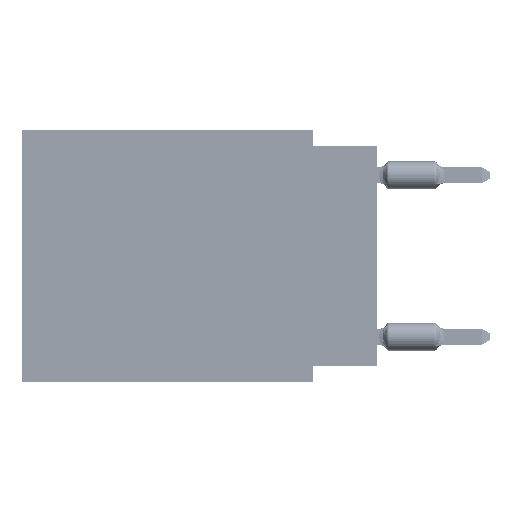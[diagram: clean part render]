
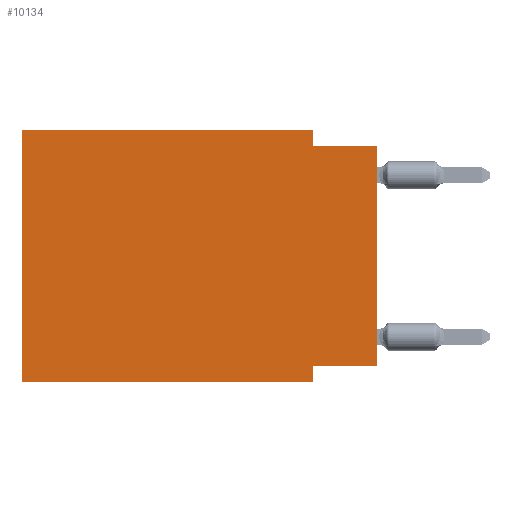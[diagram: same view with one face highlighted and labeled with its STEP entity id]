
A CAD part, left-side view. The second image highlights one B-rep face of the part: STEP entity #10134.
In plain terms, the highlighted planar face has unit normal (-1, 0, 0).
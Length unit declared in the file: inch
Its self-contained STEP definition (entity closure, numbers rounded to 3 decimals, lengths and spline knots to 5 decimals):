
#386 = CARTESIAN_POINT ( 'NONE',  ( 0., 0., -0.365 ) ) ;
#2029 = CARTESIAN_POINT ( 'NONE',  ( 0., 0.1, -0.365 ) ) ;
#3351 = PLANE ( 'NONE',  #41891 ) ;
#4363 = EDGE_CURVE ( 'NONE', #35764, #25102, #34389, .T. ) ;
#5950 = VERTEX_POINT ( 'NONE', #2029 ) ;
#7234 = VECTOR ( 'NONE', #46961, 39.37008 ) ;
#8746 = VECTOR ( 'NONE', #32876, 39.37008 ) ;
#9327 = CARTESIAN_POINT ( 'NONE',  ( 0., 0., -0.365 ) ) ;
#10134 = ADVANCED_FACE ( 'NONE', ( #15335 ), #3351, .F. ) ;
#11684 = VECTOR ( 'NONE', #74035, 39.37008 ) ;
#11766 = DIRECTION ( 'NONE',  ( 0., 0., -1. ) ) ;
#11828 = ORIENTED_EDGE ( 'NONE', *, *, #55855, .T. ) ;
#11961 = VECTOR ( 'NONE', #77075, 39.37008 ) ;
#12108 = LINE ( 'NONE', #53557, #12975 ) ;
#12199 = VERTEX_POINT ( 'NONE', #55773 ) ;
#12975 = VECTOR ( 'NONE', #66747, 39.37008 ) ;
#15335 = FACE_OUTER_BOUND ( 'NONE', #48229, .T. ) ;
#18091 = ORIENTED_EDGE ( 'NONE', *, *, #24959, .F. ) ;
#18726 = VECTOR ( 'NONE', #11766, 39.37008 ) ;
#18885 = ORIENTED_EDGE ( 'NONE', *, *, #45649, .F. ) ;
#20307 = ORIENTED_EDGE ( 'NONE', *, *, #33923, .F. ) ;
#20391 = DIRECTION ( 'NONE',  ( 0., 0., 1. ) ) ;
#21571 = VERTEX_POINT ( 'NONE', #386 ) ;
#21689 = DIRECTION ( 'NONE',  ( 1., 0., 0. ) ) ;
#21974 = CARTESIAN_POINT ( 'NONE',  ( 0., 0.55, -0.39 ) ) ;
#24959 = EDGE_CURVE ( 'NONE', #42653, #35764, #12108, .T. ) ;
#25102 = VERTEX_POINT ( 'NONE', #68686 ) ;
#25764 = CARTESIAN_POINT ( 'NONE',  ( 0., 0.55, -0.39 ) ) ;
#26309 = CARTESIAN_POINT ( 'NONE',  ( 0., 0.55, 0. ) ) ;
#26768 = CARTESIAN_POINT ( 'NONE',  ( 0., 0.55, 0. ) ) ;
#28145 = VERTEX_POINT ( 'NONE', #70211 ) ;
#28899 = LINE ( 'NONE', #48055, #18726 ) ;
#32876 = DIRECTION ( 'NONE',  ( 0., 1., 0. ) ) ;
#33552 = LINE ( 'NONE', #26768, #55166 ) ;
#33923 = EDGE_CURVE ( 'NONE', #25102, #12199, #64913, .T. ) ;
#34389 = LINE ( 'NONE', #54301, #11961 ) ;
#34483 = EDGE_CURVE ( 'NONE', #5950, #28145, #28899, .T. ) ;
#34598 = CARTESIAN_POINT ( 'NONE',  ( 0., 0., -0.025 ) ) ;
#35478 = LINE ( 'NONE', #48240, #49902 ) ;
#35764 = VERTEX_POINT ( 'NONE', #76562 ) ;
#39154 = ORIENTED_EDGE ( 'NONE', *, *, #34483, .F. ) ;
#39558 = ORIENTED_EDGE ( 'NONE', *, *, #43475, .T. ) ;
#41891 = AXIS2_PLACEMENT_3D ( 'NONE', #76345, #21689, #46039 ) ;
#42653 = VERTEX_POINT ( 'NONE', #26309 ) ;
#43475 = EDGE_CURVE ( 'NONE', #72529, #28145, #56857, .T. ) ;
#45649 = EDGE_CURVE ( 'NONE', #72529, #42653, #33552, .T. ) ;
#46039 = DIRECTION ( 'NONE',  ( 0., 0., -1. ) ) ;
#46961 = DIRECTION ( 'NONE',  ( 0., -1., 0. ) ) ;
#47443 = DIRECTION ( 'NONE',  ( 0., 0., 1. ) ) ;
#48055 = CARTESIAN_POINT ( 'NONE',  ( 0., 0.1, -0.39 ) ) ;
#48229 = EDGE_LOOP ( 'NONE', ( #11828, #20307, #75558, #18091, #18885, #39558, #39154, #71992 ) ) ;
#48240 = CARTESIAN_POINT ( 'NONE',  ( 0., 0., 0. ) ) ;
#49902 = VECTOR ( 'NONE', #47443, 39.37008 ) ;
#53557 = CARTESIAN_POINT ( 'NONE',  ( 0., 0.55, 0. ) ) ;
#54301 = CARTESIAN_POINT ( 'NONE',  ( 0., 0.1, 0. ) ) ;
#55166 = VECTOR ( 'NONE', #20391, 39.37008 ) ;
#55773 = CARTESIAN_POINT ( 'NONE',  ( 0., 0., -0.025 ) ) ;
#55855 = EDGE_CURVE ( 'NONE', #21571, #12199, #35478, .T. ) ;
#56857 = LINE ( 'NONE', #25764, #11684 ) ;
#64913 = LINE ( 'NONE', #34598, #7234 ) ;
#66747 = DIRECTION ( 'NONE',  ( 0., -1., 0. ) ) ;
#68686 = CARTESIAN_POINT ( 'NONE',  ( 0., 0.1, -0.025 ) ) ;
#69575 = LINE ( 'NONE', #9327, #8746 ) ;
#70211 = CARTESIAN_POINT ( 'NONE',  ( 0., 0.1, -0.39 ) ) ;
#71992 = ORIENTED_EDGE ( 'NONE', *, *, #77746, .F. ) ;
#72529 = VERTEX_POINT ( 'NONE', #21974 ) ;
#74035 = DIRECTION ( 'NONE',  ( 0., -1., 0. ) ) ;
#75558 = ORIENTED_EDGE ( 'NONE', *, *, #4363, .F. ) ;
#76345 = CARTESIAN_POINT ( 'NONE',  ( 0., 0.55, 0. ) ) ;
#76562 = CARTESIAN_POINT ( 'NONE',  ( 0., 0.1, 0. ) ) ;
#77075 = DIRECTION ( 'NONE',  ( 0., 0., -1. ) ) ;
#77746 = EDGE_CURVE ( 'NONE', #21571, #5950, #69575, .T. ) ;
